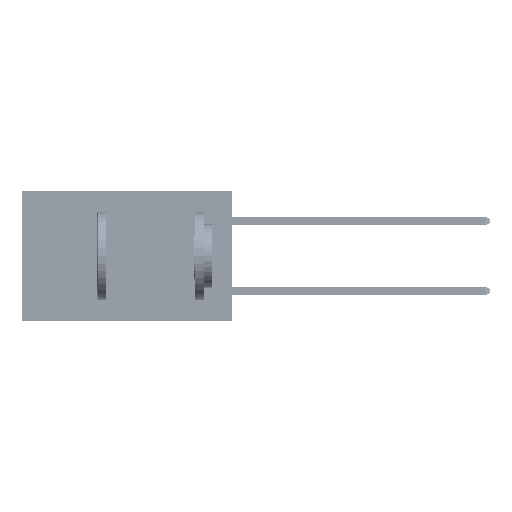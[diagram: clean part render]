
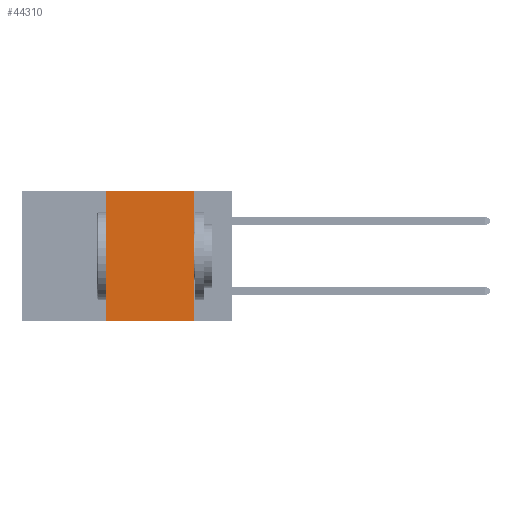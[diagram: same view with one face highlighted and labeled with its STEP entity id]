
A CAD part, left-side view. The second image highlights one B-rep face of the part: STEP entity #44310.
In plain terms, the highlighted planar face has unit normal (-1, 0, 0).
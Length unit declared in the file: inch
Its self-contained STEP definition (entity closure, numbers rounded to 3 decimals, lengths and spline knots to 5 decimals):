
#2107 = ORIENTED_EDGE ( 'NONE', *, *, #29767, .F. ) ;
#2923 = PLANE ( 'NONE',  #35923 ) ;
#4101 = VERTEX_POINT ( 'NONE', #23794 ) ;
#4927 = CARTESIAN_POINT ( 'NONE',  ( 0., 0.36, 0. ) ) ;
#5918 = LINE ( 'NONE', #36550, #26558 ) ;
#6517 = EDGE_LOOP ( 'NONE', ( #45752, #51419, #2107, #45693 ) ) ;
#8637 = VERTEX_POINT ( 'NONE', #4927 ) ;
#8694 = DIRECTION ( 'NONE',  ( 0., 0., -1. ) ) ;
#11293 = CARTESIAN_POINT ( 'NONE',  ( 0., 0.6, 0. ) ) ;
#13039 = CARTESIAN_POINT ( 'NONE',  ( 0., 0.11, -0.37 ) ) ;
#14317 = EDGE_CURVE ( 'NONE', #30166, #29092, #21223, .T. ) ;
#15459 = DIRECTION ( 'NONE',  ( 0., 0., -1. ) ) ;
#16239 = VECTOR ( 'NONE', #25606, 39.37008 ) ;
#19670 = CARTESIAN_POINT ( 'NONE',  ( 0., 0.6, -0.37 ) ) ;
#20101 = FACE_OUTER_BOUND ( 'NONE', #6517, .T. ) ;
#20412 = DIRECTION ( 'NONE',  ( 0., -1., 0. ) ) ;
#21223 = LINE ( 'NONE', #19670, #30738 ) ;
#23747 = EDGE_CURVE ( 'NONE', #4101, #29092, #50080, .T. ) ;
#23794 = CARTESIAN_POINT ( 'NONE',  ( 0., 0.11, 0. ) ) ;
#25606 = DIRECTION ( 'NONE',  ( 0., 0., 1. ) ) ;
#26558 = VECTOR ( 'NONE', #20412, 39.37008 ) ;
#28062 = CARTESIAN_POINT ( 'NONE',  ( 0., 0.36, -0.37 ) ) ;
#28552 = VECTOR ( 'NONE', #8694, 39.37008 ) ;
#29092 = VERTEX_POINT ( 'NONE', #13039 ) ;
#29767 = EDGE_CURVE ( 'NONE', #30166, #8637, #32315, .T. ) ;
#30166 = VERTEX_POINT ( 'NONE', #28062 ) ;
#30738 = VECTOR ( 'NONE', #31938, 39.37008 ) ;
#31938 = DIRECTION ( 'NONE',  ( 0., -1., 0. ) ) ;
#32315 = LINE ( 'NONE', #33705, #16239 ) ;
#33705 = CARTESIAN_POINT ( 'NONE',  ( 0., 0.36, 0. ) ) ;
#35923 = AXIS2_PLACEMENT_3D ( 'NONE', #11293, #39886, #15459 ) ;
#36550 = CARTESIAN_POINT ( 'NONE',  ( 0., 0.6, 0. ) ) ;
#39886 = DIRECTION ( 'NONE',  ( 1., 0., 0. ) ) ;
#41381 = CARTESIAN_POINT ( 'NONE',  ( 0., 0.11, 0. ) ) ;
#43736 = EDGE_CURVE ( 'NONE', #8637, #4101, #5918, .T. ) ;
#44310 = ADVANCED_FACE ( 'NONE', ( #20101 ), #2923, .F. ) ;
#45693 = ORIENTED_EDGE ( 'NONE', *, *, #14317, .T. ) ;
#45752 = ORIENTED_EDGE ( 'NONE', *, *, #23747, .F. ) ;
#50080 = LINE ( 'NONE', #41381, #28552 ) ;
#51419 = ORIENTED_EDGE ( 'NONE', *, *, #43736, .F. ) ;
